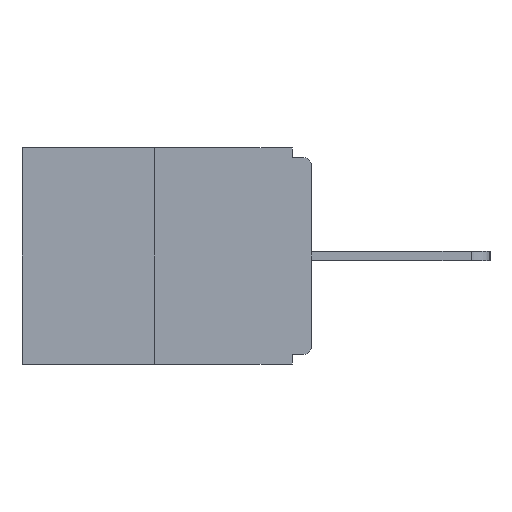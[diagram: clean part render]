
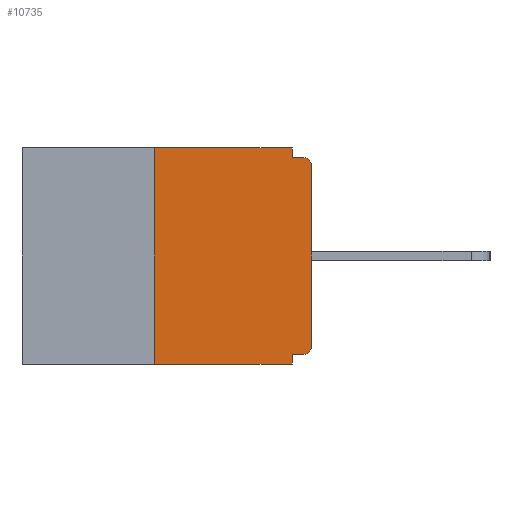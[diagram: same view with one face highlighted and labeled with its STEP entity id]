
A CAD part, left-side view. The second image highlights one B-rep face of the part: STEP entity #10735.
In plain terms, the highlighted planar face has unit normal (-1, 0, 0).
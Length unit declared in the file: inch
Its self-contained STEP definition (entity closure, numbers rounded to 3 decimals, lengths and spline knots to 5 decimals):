
#1136 = LINE ( 'NONE', #4903, #11516 ) ;
#1203 = DIRECTION ( 'NONE',  ( 1., 0., 0. ) ) ;
#1292 = ORIENTED_EDGE ( 'NONE', *, *, #3634, .F. ) ;
#1412 = DIRECTION ( 'NONE',  ( 0., 0., -1. ) ) ;
#1679 = EDGE_CURVE ( 'NONE', #12295, #11595, #6372, .T. ) ;
#1872 = VECTOR ( 'NONE', #12770, 39.37008 ) ;
#1940 = ORIENTED_EDGE ( 'NONE', *, *, #7640, .F. ) ;
#1945 = CARTESIAN_POINT ( 'NONE',  ( 0., 0.46, -0.343 ) ) ;
#1970 = VERTEX_POINT ( 'NONE', #8832 ) ;
#2654 = CIRCLE ( 'NONE', #6139, 0.015 ) ;
#2721 = CARTESIAN_POINT ( 'NONE',  ( 0., 0., -0.015 ) ) ;
#2774 = ORIENTED_EDGE ( 'NONE', *, *, #16287, .T. ) ;
#3033 = LINE ( 'NONE', #5623, #15495 ) ;
#3285 = ORIENTED_EDGE ( 'NONE', *, *, #8864, .T. ) ;
#3470 = CIRCLE ( 'NONE', #11959, 0.015 ) ;
#3563 = PLANE ( 'NONE',  #13864 ) ;
#3634 = EDGE_CURVE ( 'NONE', #14243, #4038, #1136, .T. ) ;
#3763 = LINE ( 'NONE', #10175, #9818 ) ;
#4038 = VERTEX_POINT ( 'NONE', #7566 ) ;
#4515 = VERTEX_POINT ( 'NONE', #7619 ) ;
#4646 = CARTESIAN_POINT ( 'NONE',  ( 0., 0.015, -0.313 ) ) ;
#4673 = EDGE_LOOP ( 'NONE', ( #1292, #7176, #2774, #15617, #9023, #14987, #11125, #3285, #9771, #1940 ) ) ;
#4739 = LINE ( 'NONE', #10802, #5554 ) ;
#4903 = CARTESIAN_POINT ( 'NONE',  ( 0., 0.46, 0. ) ) ;
#5554 = VECTOR ( 'NONE', #16096, 39.37008 ) ;
#5623 = CARTESIAN_POINT ( 'NONE',  ( 0., 0.25, 0. ) ) ;
#6139 = AXIS2_PLACEMENT_3D ( 'NONE', #4646, #9643, #12108 ) ;
#6256 = CARTESIAN_POINT ( 'NONE',  ( 0., 0.46, 0. ) ) ;
#6370 = DIRECTION ( 'NONE',  ( 0., 0., -1. ) ) ;
#6372 = LINE ( 'NONE', #16221, #10653 ) ;
#6472 = VERTEX_POINT ( 'NONE', #13122 ) ;
#7176 = ORIENTED_EDGE ( 'NONE', *, *, #11522, .F. ) ;
#7488 = DIRECTION ( 'NONE',  ( 0., 0., -1. ) ) ;
#7566 = CARTESIAN_POINT ( 'NONE',  ( 0., 0.031, 0. ) ) ;
#7574 = EDGE_CURVE ( 'NONE', #14091, #6472, #15048, .T. ) ;
#7575 = FACE_OUTER_BOUND ( 'NONE', #4673, .T. ) ;
#7619 = CARTESIAN_POINT ( 'NONE',  ( 0., 0.015, -0.328 ) ) ;
#7640 = EDGE_CURVE ( 'NONE', #4038, #16374, #3763, .T. ) ;
#8263 = EDGE_CURVE ( 'NONE', #4515, #12295, #2654, .T. ) ;
#8832 = CARTESIAN_POINT ( 'NONE',  ( 0., 0.25, -0.343 ) ) ;
#8864 = EDGE_CURVE ( 'NONE', #11595, #14305, #3470, .T. ) ;
#9023 = ORIENTED_EDGE ( 'NONE', *, *, #15323, .F. ) ;
#9444 = DIRECTION ( 'NONE',  ( 0., -1., 0. ) ) ;
#9510 = DIRECTION ( 'NONE',  ( 0., 0., 1. ) ) ;
#9643 = DIRECTION ( 'NONE',  ( -1., 0., 0. ) ) ;
#9672 = EDGE_CURVE ( 'NONE', #16374, #14305, #12681, .T. ) ;
#9771 = ORIENTED_EDGE ( 'NONE', *, *, #9672, .F. ) ;
#9818 = VECTOR ( 'NONE', #1412, 39.37008 ) ;
#10112 = DIRECTION ( 'NONE',  ( 0., 0., -1. ) ) ;
#10175 = CARTESIAN_POINT ( 'NONE',  ( 0., 0.031, 0. ) ) ;
#10257 = DIRECTION ( 'NONE',  ( 0., 0., 1. ) ) ;
#10653 = VECTOR ( 'NONE', #10257, 39.37008 ) ;
#10690 = LINE ( 'NONE', #1945, #12932 ) ;
#10735 = ADVANCED_FACE ( 'NONE', ( #7575 ), #3563, .F. ) ;
#10802 = CARTESIAN_POINT ( 'NONE',  ( 0., 0., -0.328 ) ) ;
#11125 = ORIENTED_EDGE ( 'NONE', *, *, #1679, .T. ) ;
#11294 = CARTESIAN_POINT ( 'NONE',  ( 0., 0.25, 0. ) ) ;
#11516 = VECTOR ( 'NONE', #12357, 39.37008 ) ;
#11522 = EDGE_CURVE ( 'NONE', #1970, #14243, #3033, .T. ) ;
#11595 = VERTEX_POINT ( 'NONE', #13718 ) ;
#11619 = CARTESIAN_POINT ( 'NONE',  ( 0., 0.015, -0.015 ) ) ;
#11959 = AXIS2_PLACEMENT_3D ( 'NONE', #14925, #12333, #10112 ) ;
#12108 = DIRECTION ( 'NONE',  ( 0., 0., -1. ) ) ;
#12295 = VERTEX_POINT ( 'NONE', #15463 ) ;
#12333 = DIRECTION ( 'NONE',  ( -1., 0., 0. ) ) ;
#12357 = DIRECTION ( 'NONE',  ( 0., -1., 0. ) ) ;
#12681 = LINE ( 'NONE', #2721, #1872 ) ;
#12770 = DIRECTION ( 'NONE',  ( 0., -1., 0. ) ) ;
#12932 = VECTOR ( 'NONE', #9444, 39.37008 ) ;
#13122 = CARTESIAN_POINT ( 'NONE',  ( 0., 0.031, -0.343 ) ) ;
#13718 = CARTESIAN_POINT ( 'NONE',  ( 0., 0., -0.03 ) ) ;
#13864 = AXIS2_PLACEMENT_3D ( 'NONE', #6256, #1203, #7488 ) ;
#14091 = VERTEX_POINT ( 'NONE', #14775 ) ;
#14243 = VERTEX_POINT ( 'NONE', #11294 ) ;
#14305 = VERTEX_POINT ( 'NONE', #11619 ) ;
#14775 = CARTESIAN_POINT ( 'NONE',  ( 0., 0.031, -0.328 ) ) ;
#14839 = VECTOR ( 'NONE', #6370, 39.37008 ) ;
#14925 = CARTESIAN_POINT ( 'NONE',  ( 0., 0.015, -0.03 ) ) ;
#14987 = ORIENTED_EDGE ( 'NONE', *, *, #8263, .T. ) ;
#15048 = LINE ( 'NONE', #16302, #14839 ) ;
#15323 = EDGE_CURVE ( 'NONE', #4515, #14091, #4739, .T. ) ;
#15463 = CARTESIAN_POINT ( 'NONE',  ( 0., 0., -0.313 ) ) ;
#15495 = VECTOR ( 'NONE', #9510, 39.37008 ) ;
#15617 = ORIENTED_EDGE ( 'NONE', *, *, #7574, .F. ) ;
#16096 = DIRECTION ( 'NONE',  ( 0., 1., 0. ) ) ;
#16142 = CARTESIAN_POINT ( 'NONE',  ( 0., 0.031, -0.015 ) ) ;
#16221 = CARTESIAN_POINT ( 'NONE',  ( 0., 0., 0. ) ) ;
#16287 = EDGE_CURVE ( 'NONE', #1970, #6472, #10690, .T. ) ;
#16302 = CARTESIAN_POINT ( 'NONE',  ( 0., 0.031, -0.343 ) ) ;
#16374 = VERTEX_POINT ( 'NONE', #16142 ) ;
